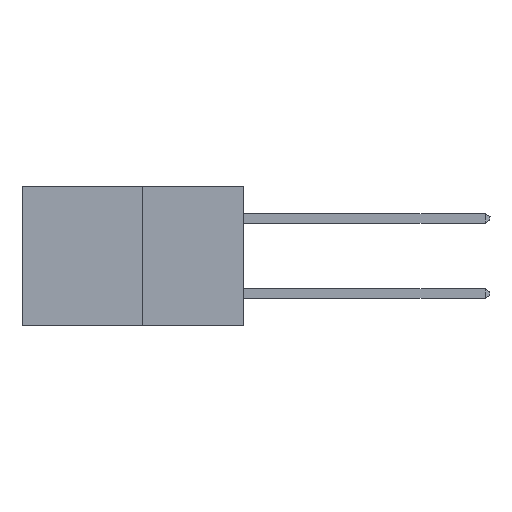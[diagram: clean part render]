
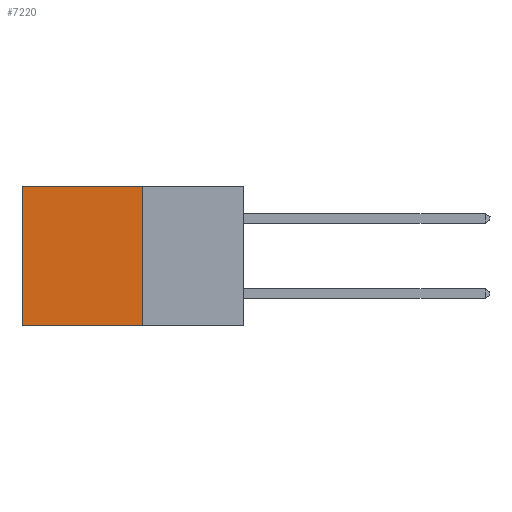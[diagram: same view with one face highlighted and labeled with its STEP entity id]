
A CAD part, left-side view. The second image highlights one B-rep face of the part: STEP entity #7220.
In plain terms, the highlighted planar face has unit normal (-1, 0, 0).
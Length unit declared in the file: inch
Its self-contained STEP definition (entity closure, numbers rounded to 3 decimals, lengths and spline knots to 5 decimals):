
#407 = VERTEX_POINT ( 'NONE', #6198 ) ;
#647 = LINE ( 'NONE', #13288, #6019 ) ;
#881 = DIRECTION ( 'NONE',  ( 0., 0., -1. ) ) ;
#1081 = EDGE_CURVE ( 'NONE', #10012, #3711, #6043, .T. ) ;
#1304 = ORIENTED_EDGE ( 'NONE', *, *, #11352, .F. ) ;
#1976 = CARTESIAN_POINT ( 'NONE',  ( 0.277, 0.59, -0.37 ) ) ;
#2720 = EDGE_CURVE ( 'NONE', #407, #13291, #647, .T. ) ;
#2902 = VECTOR ( 'NONE', #11348, 39.37008 ) ;
#3167 = ORIENTED_EDGE ( 'NONE', *, *, #1081, .F. ) ;
#3518 = CARTESIAN_POINT ( 'NONE',  ( 0.277, 0.27, -0.37 ) ) ;
#3711 = VERTEX_POINT ( 'NONE', #1976 ) ;
#3782 = ORIENTED_EDGE ( 'NONE', *, *, #2720, .T. ) ;
#4048 = ORIENTED_EDGE ( 'NONE', *, *, #4863, .T. ) ;
#4639 = LINE ( 'NONE', #13260, #12583 ) ;
#4735 = LINE ( 'NONE', #13394, #13009 ) ;
#4863 = EDGE_CURVE ( 'NONE', #13291, #3711, #4735, .T. ) ;
#5799 = FACE_OUTER_BOUND ( 'NONE', #10765, .T. ) ;
#6019 = VECTOR ( 'NONE', #13252, 39.37008 ) ;
#6043 = LINE ( 'NONE', #3518, #2902 ) ;
#6089 = DIRECTION ( 'NONE',  ( 0., 0., -1. ) ) ;
#6122 = DIRECTION ( 'NONE',  ( 1., 0., 0. ) ) ;
#6174 = PLANE ( 'NONE',  #11013 ) ;
#6198 = CARTESIAN_POINT ( 'NONE',  ( 0.277, 0.27, 0. ) ) ;
#6202 = CARTESIAN_POINT ( 'NONE',  ( 0.277, 0.27, -0.37 ) ) ;
#7119 = CARTESIAN_POINT ( 'NONE',  ( 0.277, 0.27, -0.37 ) ) ;
#7220 = ADVANCED_FACE ( 'NONE', ( #5799 ), #6174, .F. ) ;
#10012 = VERTEX_POINT ( 'NONE', #7119 ) ;
#10187 = DIRECTION ( 'NONE',  ( 0., 0., -1. ) ) ;
#10706 = CARTESIAN_POINT ( 'NONE',  ( 0.277, 0.59, 0. ) ) ;
#10765 = EDGE_LOOP ( 'NONE', ( #4048, #3167, #1304, #3782 ) ) ;
#11013 = AXIS2_PLACEMENT_3D ( 'NONE', #6202, #6122, #6089 ) ;
#11348 = DIRECTION ( 'NONE',  ( 0., 1., 0. ) ) ;
#11352 = EDGE_CURVE ( 'NONE', #407, #10012, #4639, .T. ) ;
#12583 = VECTOR ( 'NONE', #10187, 39.37008 ) ;
#13009 = VECTOR ( 'NONE', #881, 39.37008 ) ;
#13252 = DIRECTION ( 'NONE',  ( 0., 1., 0. ) ) ;
#13260 = CARTESIAN_POINT ( 'NONE',  ( 0.277, 0.27, -0.37 ) ) ;
#13288 = CARTESIAN_POINT ( 'NONE',  ( 0.277, 0.27, 0. ) ) ;
#13291 = VERTEX_POINT ( 'NONE', #10706 ) ;
#13394 = CARTESIAN_POINT ( 'NONE',  ( 0.277, 0.59, -0.37 ) ) ;
